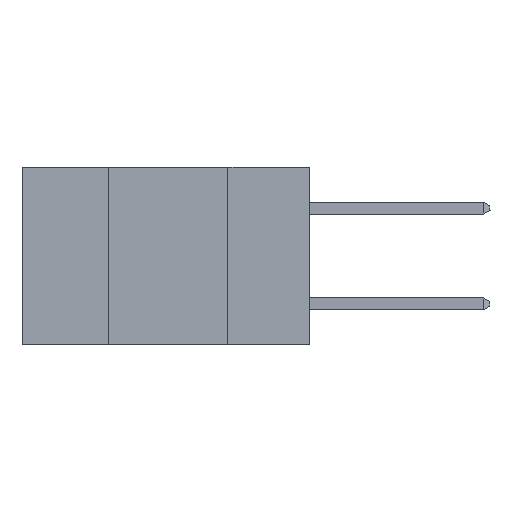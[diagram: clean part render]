
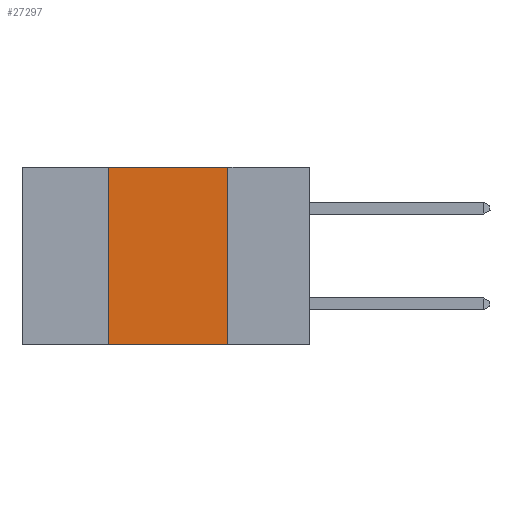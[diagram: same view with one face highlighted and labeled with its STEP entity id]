
A CAD part, left-side view. The second image highlights one B-rep face of the part: STEP entity #27297.
In plain terms, the highlighted planar face has unit normal (-1, 0, 0).
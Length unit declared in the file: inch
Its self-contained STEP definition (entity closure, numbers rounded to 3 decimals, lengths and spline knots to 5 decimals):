
#980 = DIRECTION ( 'NONE',  ( 0., -1., 0. ) ) ;
#2060 = LINE ( 'NONE', #27608, #21062 ) ;
#2790 = VECTOR ( 'NONE', #25574, 39.37008 ) ;
#3272 = DIRECTION ( 'NONE',  ( 0., -1., 0. ) ) ;
#3354 = EDGE_CURVE ( 'NONE', #22843, #11660, #16304, .T. ) ;
#3557 = ORIENTED_EDGE ( 'NONE', *, *, #4737, .T. ) ;
#4737 = EDGE_CURVE ( 'NONE', #22843, #16453, #7352, .T. ) ;
#6954 = VERTEX_POINT ( 'NONE', #32372 ) ;
#7352 = LINE ( 'NONE', #22396, #33674 ) ;
#7407 = PLANE ( 'NONE',  #20766 ) ;
#7880 = VECTOR ( 'NONE', #3272, 39.37008 ) ;
#8054 = ORIENTED_EDGE ( 'NONE', *, *, #36856, .F. ) ;
#9005 = CARTESIAN_POINT ( 'NONE',  ( 0., 0.42, -0.37 ) ) ;
#9604 = CARTESIAN_POINT ( 'NONE',  ( 0., 0.42, 0. ) ) ;
#10895 = DIRECTION ( 'NONE',  ( 0., 0., -1. ) ) ;
#11660 = VERTEX_POINT ( 'NONE', #9604 ) ;
#13474 = ORIENTED_EDGE ( 'NONE', *, *, #34410, .F. ) ;
#14204 = DIRECTION ( 'NONE',  ( 0., 0., -1. ) ) ;
#16304 = LINE ( 'NONE', #26187, #2790 ) ;
#16453 = VERTEX_POINT ( 'NONE', #31364 ) ;
#19564 = CARTESIAN_POINT ( 'NONE',  ( 0., 0.6, 0. ) ) ;
#19762 = ORIENTED_EDGE ( 'NONE', *, *, #3354, .F. ) ;
#20477 = CARTESIAN_POINT ( 'NONE',  ( 0., 0.6, 0. ) ) ;
#20766 = AXIS2_PLACEMENT_3D ( 'NONE', #19564, #23257, #10895 ) ;
#21062 = VECTOR ( 'NONE', #14204, 39.37008 ) ;
#22396 = CARTESIAN_POINT ( 'NONE',  ( 0., 0.6, -0.37 ) ) ;
#22843 = VERTEX_POINT ( 'NONE', #9005 ) ;
#23257 = DIRECTION ( 'NONE',  ( 1., 0., 0. ) ) ;
#25281 = LINE ( 'NONE', #20477, #7880 ) ;
#25574 = DIRECTION ( 'NONE',  ( 0., 0., 1. ) ) ;
#25940 = FACE_OUTER_BOUND ( 'NONE', #40213, .T. ) ;
#26187 = CARTESIAN_POINT ( 'NONE',  ( 0., 0.42, 0. ) ) ;
#27297 = ADVANCED_FACE ( 'NONE', ( #25940 ), #7407, .F. ) ;
#27608 = CARTESIAN_POINT ( 'NONE',  ( 0., 0.17, 0. ) ) ;
#31364 = CARTESIAN_POINT ( 'NONE',  ( 0., 0.17, -0.37 ) ) ;
#32372 = CARTESIAN_POINT ( 'NONE',  ( 0., 0.17, 0. ) ) ;
#33674 = VECTOR ( 'NONE', #980, 39.37008 ) ;
#34410 = EDGE_CURVE ( 'NONE', #11660, #6954, #25281, .T. ) ;
#36856 = EDGE_CURVE ( 'NONE', #6954, #16453, #2060, .T. ) ;
#40213 = EDGE_LOOP ( 'NONE', ( #8054, #13474, #19762, #3557 ) ) ;
